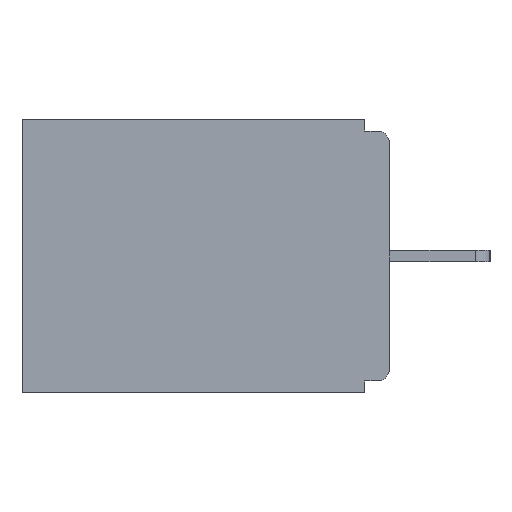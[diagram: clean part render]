
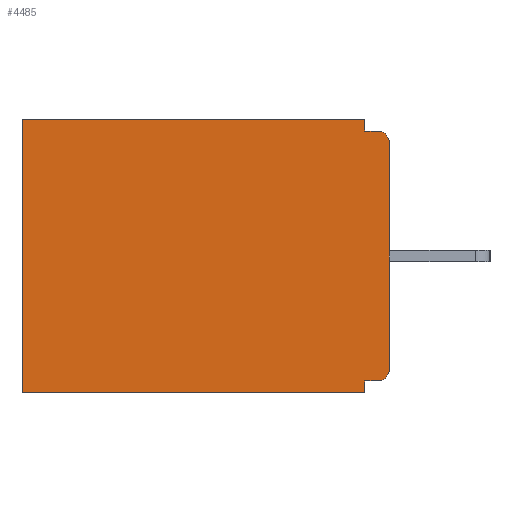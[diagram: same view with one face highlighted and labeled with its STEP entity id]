
A CAD part, left-side view. The second image highlights one B-rep face of the part: STEP entity #4485.
In plain terms, the highlighted planar face has unit normal (-1, 0, 0).
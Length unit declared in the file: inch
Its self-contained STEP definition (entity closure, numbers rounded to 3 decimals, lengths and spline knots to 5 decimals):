
#213 = VECTOR ( 'NONE', #9301, 39.37008 ) ;
#303 = VERTEX_POINT ( 'NONE', #15966 ) ;
#656 = CARTESIAN_POINT ( 'NONE',  ( 0.298, 0.015, -0.03 ) ) ;
#754 = CARTESIAN_POINT ( 'NONE',  ( 0.298, 0., 0. ) ) ;
#1359 = EDGE_CURVE ( 'NONE', #7645, #13316, #12903, .T. ) ;
#1524 = VECTOR ( 'NONE', #8295, 39.37008 ) ;
#1815 = DIRECTION ( 'NONE',  ( 0., 1., 0. ) ) ;
#1886 = CARTESIAN_POINT ( 'NONE',  ( 0.298, 0.015, -0.313 ) ) ;
#2244 = CARTESIAN_POINT ( 'NONE',  ( 0.298, 0.46, -0.343 ) ) ;
#2350 = LINE ( 'NONE', #6780, #12774 ) ;
#2375 = VECTOR ( 'NONE', #16480, 39.37008 ) ;
#2621 = EDGE_CURVE ( 'NONE', #16282, #5093, #4998, .T. ) ;
#2639 = CARTESIAN_POINT ( 'NONE',  ( 0.298, 0., 0. ) ) ;
#2890 = EDGE_CURVE ( 'NONE', #16280, #13573, #9394, .T. ) ;
#2933 = VERTEX_POINT ( 'NONE', #8559 ) ;
#3033 = DIRECTION ( 'NONE',  ( 0., 0., -1. ) ) ;
#3241 = ORIENTED_EDGE ( 'NONE', *, *, #14062, .F. ) ;
#3560 = AXIS2_PLACEMENT_3D ( 'NONE', #1886, #8523, #7421 ) ;
#3841 = CIRCLE ( 'NONE', #17212, 0.015 ) ;
#3990 = VECTOR ( 'NONE', #10622, 39.37008 ) ;
#4333 = ORIENTED_EDGE ( 'NONE', *, *, #6035, .T. ) ;
#4359 = DIRECTION ( 'NONE',  ( -1., 0., 0. ) ) ;
#4485 = ADVANCED_FACE ( 'NONE', ( #8266 ), #17982, .F. ) ;
#4599 = CARTESIAN_POINT ( 'NONE',  ( 0.298, 0., -0.328 ) ) ;
#4998 = LINE ( 'NONE', #9204, #10746 ) ;
#5093 = VERTEX_POINT ( 'NONE', #11149 ) ;
#5824 = EDGE_CURVE ( 'NONE', #13316, #16280, #11019, .T. ) ;
#5857 = ORIENTED_EDGE ( 'NONE', *, *, #14638, .F. ) ;
#6035 = EDGE_CURVE ( 'NONE', #14875, #5093, #3841, .T. ) ;
#6780 = CARTESIAN_POINT ( 'NONE',  ( 0.298, 0., 0. ) ) ;
#7421 = DIRECTION ( 'NONE',  ( 0., 0., -1. ) ) ;
#7645 = VERTEX_POINT ( 'NONE', #7705 ) ;
#7654 = LINE ( 'NONE', #754, #213 ) ;
#7705 = CARTESIAN_POINT ( 'NONE',  ( 0.298, 0.015, -0.328 ) ) ;
#7895 = CARTESIAN_POINT ( 'NONE',  ( 0.298, 0.031, -0.328 ) ) ;
#8055 = EDGE_CURVE ( 'NONE', #7645, #14715, #9079, .T. ) ;
#8243 = DIRECTION ( 'NONE',  ( 0., 1., 0. ) ) ;
#8266 = FACE_OUTER_BOUND ( 'NONE', #14710, .T. ) ;
#8295 = DIRECTION ( 'NONE',  ( 0., 0., -1. ) ) ;
#8523 = DIRECTION ( 'NONE',  ( -1., 0., 0. ) ) ;
#8559 = CARTESIAN_POINT ( 'NONE',  ( 0.298, 0.031, 0. ) ) ;
#9079 = CIRCLE ( 'NONE', #3560, 0.015 ) ;
#9204 = CARTESIAN_POINT ( 'NONE',  ( 0.298, 0., -0.015 ) ) ;
#9301 = DIRECTION ( 'NONE',  ( 0., 0., -1. ) ) ;
#9394 = LINE ( 'NONE', #14936, #2375 ) ;
#9635 = CARTESIAN_POINT ( 'NONE',  ( 0.298, 0.031, -0.343 ) ) ;
#9671 = CARTESIAN_POINT ( 'NONE',  ( 0.298, 0.031, -0.343 ) ) ;
#10259 = CARTESIAN_POINT ( 'NONE',  ( 0.298, 0., -0.03 ) ) ;
#10556 = ORIENTED_EDGE ( 'NONE', *, *, #5824, .F. ) ;
#10615 = ORIENTED_EDGE ( 'NONE', *, *, #2621, .F. ) ;
#10622 = DIRECTION ( 'NONE',  ( 0., 0., -1. ) ) ;
#10746 = VECTOR ( 'NONE', #13118, 39.37008 ) ;
#10983 = LINE ( 'NONE', #9635, #3990 ) ;
#11019 = LINE ( 'NONE', #9671, #1524 ) ;
#11149 = CARTESIAN_POINT ( 'NONE',  ( 0.298, 0.015, -0.015 ) ) ;
#11560 = LINE ( 'NONE', #12840, #15357 ) ;
#12202 = VECTOR ( 'NONE', #1815, 39.37008 ) ;
#12255 = CARTESIAN_POINT ( 'NONE',  ( 0.298, 0.031, -0.343 ) ) ;
#12470 = ORIENTED_EDGE ( 'NONE', *, *, #1359, .F. ) ;
#12774 = VECTOR ( 'NONE', #8243, 39.37008 ) ;
#12840 = CARTESIAN_POINT ( 'NONE',  ( 0.298, 0.46, 0. ) ) ;
#12903 = LINE ( 'NONE', #4599, #12202 ) ;
#13118 = DIRECTION ( 'NONE',  ( 0., -1., 0. ) ) ;
#13316 = VERTEX_POINT ( 'NONE', #7895 ) ;
#13573 = VERTEX_POINT ( 'NONE', #2244 ) ;
#13603 = AXIS2_PLACEMENT_3D ( 'NONE', #2639, #17823, #14914 ) ;
#14062 = EDGE_CURVE ( 'NONE', #14875, #14715, #7654, .T. ) ;
#14445 = ORIENTED_EDGE ( 'NONE', *, *, #16316, .T. ) ;
#14638 = EDGE_CURVE ( 'NONE', #2933, #16282, #10983, .T. ) ;
#14710 = EDGE_LOOP ( 'NONE', ( #4333, #10615, #5857, #14445, #17899, #16180, #10556, #12470, #16985, #3241 ) ) ;
#14715 = VERTEX_POINT ( 'NONE', #15259 ) ;
#14875 = VERTEX_POINT ( 'NONE', #10259 ) ;
#14914 = DIRECTION ( 'NONE',  ( 0., 0., -1. ) ) ;
#14936 = CARTESIAN_POINT ( 'NONE',  ( 0.298, 0., -0.343 ) ) ;
#15156 = CARTESIAN_POINT ( 'NONE',  ( 0.298, 0.031, -0.015 ) ) ;
#15259 = CARTESIAN_POINT ( 'NONE',  ( 0.298, 0., -0.313 ) ) ;
#15357 = VECTOR ( 'NONE', #15471, 39.37008 ) ;
#15471 = DIRECTION ( 'NONE',  ( 0., 0., -1. ) ) ;
#15520 = EDGE_CURVE ( 'NONE', #303, #13573, #11560, .T. ) ;
#15966 = CARTESIAN_POINT ( 'NONE',  ( 0.298, 0.46, 0. ) ) ;
#16180 = ORIENTED_EDGE ( 'NONE', *, *, #2890, .F. ) ;
#16280 = VERTEX_POINT ( 'NONE', #12255 ) ;
#16282 = VERTEX_POINT ( 'NONE', #15156 ) ;
#16316 = EDGE_CURVE ( 'NONE', #2933, #303, #2350, .T. ) ;
#16480 = DIRECTION ( 'NONE',  ( 0., 1., 0. ) ) ;
#16985 = ORIENTED_EDGE ( 'NONE', *, *, #8055, .T. ) ;
#17212 = AXIS2_PLACEMENT_3D ( 'NONE', #656, #4359, #3033 ) ;
#17823 = DIRECTION ( 'NONE',  ( 1., 0., 0. ) ) ;
#17899 = ORIENTED_EDGE ( 'NONE', *, *, #15520, .T. ) ;
#17982 = PLANE ( 'NONE',  #13603 ) ;
